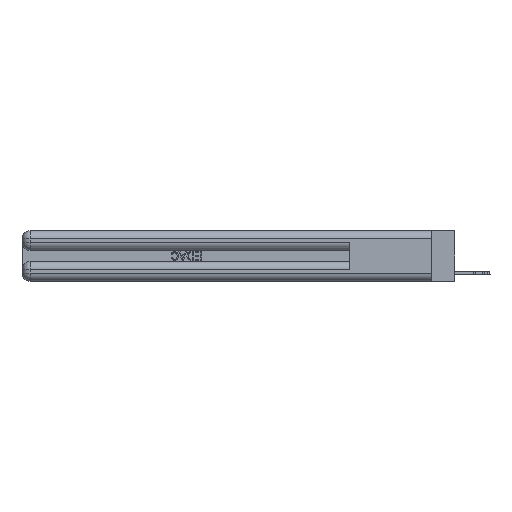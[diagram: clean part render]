
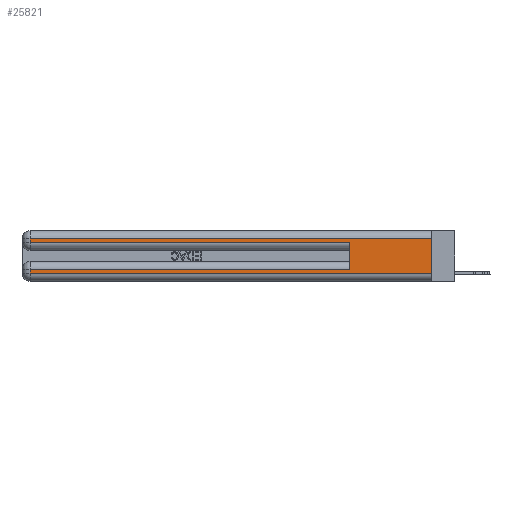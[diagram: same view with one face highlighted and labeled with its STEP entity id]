
A CAD part, left-side view. The second image highlights one B-rep face of the part: STEP entity #25821.
In plain terms, the highlighted planar face has unit normal (-1, 0, 0).
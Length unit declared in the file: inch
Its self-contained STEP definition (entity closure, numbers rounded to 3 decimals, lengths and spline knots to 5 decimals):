
#297 = LINE ( 'NONE', #10248, #15984 ) ;
#478 = LINE ( 'NONE', #1130, #27069 ) ;
#789 = CARTESIAN_POINT ( 'NONE',  ( 0., 0., 0.37 ) ) ;
#1130 = CARTESIAN_POINT ( 'NONE',  ( 0., 0., 0.37 ) ) ;
#1407 = DIRECTION ( 'NONE',  ( 0., -1., 0. ) ) ;
#1755 = DIRECTION ( 'NONE',  ( 0., 1., 0. ) ) ;
#2050 = CARTESIAN_POINT ( 'NONE',  ( 0., 2.94, 0.37 ) ) ;
#3092 = DIRECTION ( 'NONE',  ( 0., -1., 0. ) ) ;
#3275 = CARTESIAN_POINT ( 'NONE',  ( 0., 0.6, 0.085 ) ) ;
#3360 = DIRECTION ( 'NONE',  ( 0., 1., 0. ) ) ;
#3764 = VERTEX_POINT ( 'NONE', #3275 ) ;
#4494 = ORIENTED_EDGE ( 'NONE', *, *, #11239, .F. ) ;
#5376 = CARTESIAN_POINT ( 'NONE',  ( 0., 0., 0.06 ) ) ;
#5386 = CARTESIAN_POINT ( 'NONE',  ( 0., 2.94, 0.285 ) ) ;
#5476 = EDGE_CURVE ( 'NONE', #19341, #25646, #5704, .T. ) ;
#5608 = ORIENTED_EDGE ( 'NONE', *, *, #9253, .T. ) ;
#5654 = ORIENTED_EDGE ( 'NONE', *, *, #27620, .T. ) ;
#5704 = LINE ( 'NONE', #28955, #9018 ) ;
#6570 = VERTEX_POINT ( 'NONE', #5386 ) ;
#7068 = CARTESIAN_POINT ( 'NONE',  ( 0., 2.94, 0.06 ) ) ;
#7331 = DIRECTION ( 'NONE',  ( 0., 0., -1. ) ) ;
#8209 = EDGE_CURVE ( 'NONE', #22699, #19341, #297, .T. ) ;
#8317 = AXIS2_PLACEMENT_3D ( 'NONE', #789, #20536, #30954 ) ;
#8527 = ORIENTED_EDGE ( 'NONE', *, *, #11165, .T. ) ;
#8915 = LINE ( 'NONE', #11200, #16189 ) ;
#9018 = VECTOR ( 'NONE', #3092, 39.37008 ) ;
#9253 = EDGE_CURVE ( 'NONE', #26199, #20622, #16592, .T. ) ;
#9776 = VECTOR ( 'NONE', #1755, 39.37008 ) ;
#10248 = CARTESIAN_POINT ( 'NONE',  ( 0., 2.94, 0.37 ) ) ;
#10593 = FACE_OUTER_BOUND ( 'NONE', #16242, .T. ) ;
#10814 = LINE ( 'NONE', #20767, #21880 ) ;
#10982 = ORIENTED_EDGE ( 'NONE', *, *, #26226, .T. ) ;
#11079 = PLANE ( 'NONE',  #8317 ) ;
#11165 = EDGE_CURVE ( 'NONE', #20622, #6570, #24387, .T. ) ;
#11200 = CARTESIAN_POINT ( 'NONE',  ( 0., 0., 0.285 ) ) ;
#11239 = EDGE_CURVE ( 'NONE', #3764, #14614, #10814, .T. ) ;
#12329 = ORIENTED_EDGE ( 'NONE', *, *, #25806, .F. ) ;
#12839 = LINE ( 'NONE', #17887, #22400 ) ;
#12949 = DIRECTION ( 'NONE',  ( 0., 0., 1. ) ) ;
#14614 = VERTEX_POINT ( 'NONE', #15311 ) ;
#15126 = VECTOR ( 'NONE', #24556, 39.37008 ) ;
#15311 = CARTESIAN_POINT ( 'NONE',  ( 0., 0.6, 0.285 ) ) ;
#15984 = VECTOR ( 'NONE', #7331, 39.37008 ) ;
#16189 = VECTOR ( 'NONE', #1407, 39.37008 ) ;
#16242 = EDGE_LOOP ( 'NONE', ( #12329, #5608, #8527, #5654, #4494, #10982, #20712, #31544 ) ) ;
#16592 = LINE ( 'NONE', #30939, #9776 ) ;
#17887 = CARTESIAN_POINT ( 'NONE',  ( 0., 0., 0.085 ) ) ;
#19341 = VERTEX_POINT ( 'NONE', #7068 ) ;
#20536 = DIRECTION ( 'NONE',  ( 1., 0., 0. ) ) ;
#20622 = VERTEX_POINT ( 'NONE', #25467 ) ;
#20712 = ORIENTED_EDGE ( 'NONE', *, *, #8209, .T. ) ;
#20767 = CARTESIAN_POINT ( 'NONE',  ( 0., 0.6, 0.145 ) ) ;
#21880 = VECTOR ( 'NONE', #12949, 39.37008 ) ;
#22400 = VECTOR ( 'NONE', #3360, 39.37008 ) ;
#22699 = VERTEX_POINT ( 'NONE', #27213 ) ;
#24387 = LINE ( 'NONE', #2050, #15126 ) ;
#24556 = DIRECTION ( 'NONE',  ( 0., 0., -1. ) ) ;
#25216 = CARTESIAN_POINT ( 'NONE',  ( 0., 0., 0.31 ) ) ;
#25467 = CARTESIAN_POINT ( 'NONE',  ( 0., 2.94, 0.31 ) ) ;
#25646 = VERTEX_POINT ( 'NONE', #5376 ) ;
#25806 = EDGE_CURVE ( 'NONE', #26199, #25646, #478, .T. ) ;
#25821 = ADVANCED_FACE ( 'NONE', ( #10593 ), #11079, .F. ) ;
#26199 = VERTEX_POINT ( 'NONE', #25216 ) ;
#26226 = EDGE_CURVE ( 'NONE', #3764, #22699, #12839, .T. ) ;
#27069 = VECTOR ( 'NONE', #28187, 39.37008 ) ;
#27213 = CARTESIAN_POINT ( 'NONE',  ( 0., 2.94, 0.085 ) ) ;
#27620 = EDGE_CURVE ( 'NONE', #6570, #14614, #8915, .T. ) ;
#28187 = DIRECTION ( 'NONE',  ( 0., 0., -1. ) ) ;
#28955 = CARTESIAN_POINT ( 'NONE',  ( 0., 0., 0.06 ) ) ;
#30939 = CARTESIAN_POINT ( 'NONE',  ( 0., 0., 0.31 ) ) ;
#30954 = DIRECTION ( 'NONE',  ( 0., 0., -1. ) ) ;
#31544 = ORIENTED_EDGE ( 'NONE', *, *, #5476, .T. ) ;
